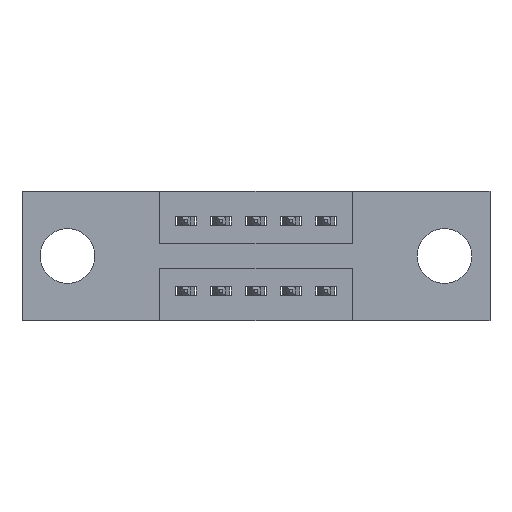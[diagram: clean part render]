
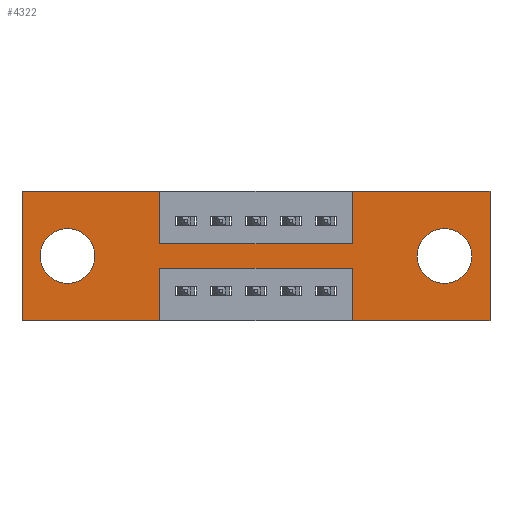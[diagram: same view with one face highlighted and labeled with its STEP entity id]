
A CAD part, front view. The second image highlights one B-rep face of the part: STEP entity #4322.
In plain terms, the highlighted planar face has unit normal (0, -1, 0).
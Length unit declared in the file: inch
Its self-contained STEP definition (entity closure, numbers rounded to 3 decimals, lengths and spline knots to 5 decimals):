
#21 = ORIENTED_EDGE ( 'NONE', *, *, #4895, .T. ) ;
#30 = CARTESIAN_POINT ( 'NONE',  ( 0.3925, 0., -0.22 ) ) ;
#129 = EDGE_CURVE ( 'NONE', #6393, #7987, #1377, .T. ) ;
#325 = CARTESIAN_POINT ( 'NONE',  ( 0.9425, 0., 0. ) ) ;
#330 = EDGE_LOOP ( 'NONE', ( #8569, #2305, #3220, #8067, #858, #7247, #7193, #8913, #1503, #1605, #1463, #5782 ) ) ;
#412 = CARTESIAN_POINT ( 'NONE',  ( 0., 0., 0. ) ) ;
#492 = CARTESIAN_POINT ( 'NONE',  ( 0.3925, 0., 0. ) ) ;
#537 = VERTEX_POINT ( 'NONE', #8299 ) ;
#549 = CARTESIAN_POINT ( 'NONE',  ( 1.205, 0., -0.185 ) ) ;
#681 = VECTOR ( 'NONE', #3747, 39.37008 ) ;
#836 = DIRECTION ( 'NONE',  ( 0., 0., 1. ) ) ;
#858 = ORIENTED_EDGE ( 'NONE', *, *, #2142, .F. ) ;
#921 = DIRECTION ( 'NONE',  ( 0., -1., 0. ) ) ;
#939 = LINE ( 'NONE', #3278, #3578 ) ;
#942 = VERTEX_POINT ( 'NONE', #8702 ) ;
#941 = CARTESIAN_POINT ( 'NONE',  ( 1.335, 0., 0. ) ) ;
#951 = VERTEX_POINT ( 'NONE', #3793 ) ;
#1284 = VERTEX_POINT ( 'NONE', #1442 ) ;
#1376 = DIRECTION ( 'NONE',  ( 0., 0., 1. ) ) ;
#1377 = CIRCLE ( 'NONE', #7139, 0.078 ) ;
#1381 = DIRECTION ( 'NONE',  ( 0., 1., 0. ) ) ;
#1442 = CARTESIAN_POINT ( 'NONE',  ( 0.3925, 0., -0.37 ) ) ;
#1462 = CARTESIAN_POINT ( 'NONE',  ( 0., 0., -0.37 ) ) ;
#1463 = ORIENTED_EDGE ( 'NONE', *, *, #4957, .F. ) ;
#1485 = CIRCLE ( 'NONE', #2098, 0.078 ) ;
#1503 = ORIENTED_EDGE ( 'NONE', *, *, #4004, .F. ) ;
#1540 = DIRECTION ( 'NONE',  ( -1., 0., 0. ) ) ;
#1567 = CARTESIAN_POINT ( 'NONE',  ( 0., 0., 0. ) ) ;
#1605 = ORIENTED_EDGE ( 'NONE', *, *, #7184, .F. ) ;
#1624 = VERTEX_POINT ( 'NONE', #7976 ) ;
#1632 = CARTESIAN_POINT ( 'NONE',  ( 0., 0., -0.37 ) ) ;
#1785 = DIRECTION ( 'NONE',  ( 0., 0., 1. ) ) ;
#1893 = VECTOR ( 'NONE', #1540, 39.37008 ) ;
#1915 = VECTOR ( 'NONE', #8106, 39.37008 ) ;
#1923 = LINE ( 'NONE', #492, #2034 ) ;
#2034 = VECTOR ( 'NONE', #3355, 39.37008 ) ;
#2061 = ORIENTED_EDGE ( 'NONE', *, *, #8958, .T. ) ;
#2098 = AXIS2_PLACEMENT_3D ( 'NONE', #549, #3452, #4260 ) ;
#2142 = EDGE_CURVE ( 'NONE', #6034, #8448, #7438, .T. ) ;
#2206 = LINE ( 'NONE', #5920, #1893 ) ;
#2228 = EDGE_CURVE ( 'NONE', #537, #8340, #939, .T. ) ;
#2305 = ORIENTED_EDGE ( 'NONE', *, *, #8248, .F. ) ;
#2360 = CIRCLE ( 'NONE', #3560, 0.078 ) ;
#2430 = LINE ( 'NONE', #7392, #681 ) ;
#2515 = VECTOR ( 'NONE', #7956, 39.37008 ) ;
#2756 = CARTESIAN_POINT ( 'NONE',  ( 0.13, 0., -0.263 ) ) ;
#2814 = VERTEX_POINT ( 'NONE', #1567 ) ;
#2815 = CARTESIAN_POINT ( 'NONE',  ( 0.13, 0., -0.185 ) ) ;
#2927 = CARTESIAN_POINT ( 'NONE',  ( 0., 0., 0. ) ) ;
#2930 = DIRECTION ( 'NONE',  ( -1., 0., 0. ) ) ;
#2950 = ORIENTED_EDGE ( 'NONE', *, *, #8917, .T. ) ;
#3128 = LINE ( 'NONE', #30, #8247 ) ;
#3137 = VECTOR ( 'NONE', #3843, 39.37008 ) ;
#3170 = CARTESIAN_POINT ( 'NONE',  ( 0.9425, 0., -0.37 ) ) ;
#3220 = ORIENTED_EDGE ( 'NONE', *, *, #8745, .F. ) ;
#3278 = CARTESIAN_POINT ( 'NONE',  ( 0.9425, 0., 0. ) ) ;
#3289 = EDGE_LOOP ( 'NONE', ( #21, #7867 ) ) ;
#3338 = FACE_BOUND ( 'NONE', #4185, .T. ) ;
#3355 = DIRECTION ( 'NONE',  ( 0., 0., -1. ) ) ;
#3452 = DIRECTION ( 'NONE',  ( 0., 1., 0. ) ) ;
#3480 = DIRECTION ( 'NONE',  ( 0., 1., 0. ) ) ;
#3560 = AXIS2_PLACEMENT_3D ( 'NONE', #2815, #5616, #4859 ) ;
#3578 = VECTOR ( 'NONE', #6212, 39.37008 ) ;
#3654 = CARTESIAN_POINT ( 'NONE',  ( 0.3925, 0., -0.15 ) ) ;
#3655 = LINE ( 'NONE', #1462, #1915 ) ;
#3747 = DIRECTION ( 'NONE',  ( 0., 0., -1. ) ) ;
#3749 = CARTESIAN_POINT ( 'NONE',  ( 1.205, 0., -0.263 ) ) ;
#3793 = CARTESIAN_POINT ( 'NONE',  ( 0.13, 0., -0.107 ) ) ;
#3843 = DIRECTION ( 'NONE',  ( 0., 0., -1. ) ) ;
#3879 = AXIS2_PLACEMENT_3D ( 'NONE', #1632, #921, #6011 ) ;
#4004 = EDGE_CURVE ( 'NONE', #7439, #4518, #1923, .T. ) ;
#4010 = VECTOR ( 'NONE', #6074, 39.37008 ) ;
#4168 = CARTESIAN_POINT ( 'NONE',  ( 1.205, 0., -0.107 ) ) ;
#4185 = EDGE_LOOP ( 'NONE', ( #2061, #2950 ) ) ;
#4260 = DIRECTION ( 'NONE',  ( 0., 0., -1. ) ) ;
#4322 = ADVANCED_FACE ( 'NONE', ( #6970, #3338, #7007 ), #8125, .T. ) ;
#4472 = EDGE_CURVE ( 'NONE', #4518, #537, #8663, .T. ) ;
#4518 = VERTEX_POINT ( 'NONE', #3654 ) ;
#4593 = EDGE_CURVE ( 'NONE', #942, #1284, #2430, .T. ) ;
#4692 = LINE ( 'NONE', #412, #4010 ) ;
#4778 = CIRCLE ( 'NONE', #5235, 0.078 ) ;
#4821 = DIRECTION ( 'NONE',  ( 1., 0., 0. ) ) ;
#4859 = DIRECTION ( 'NONE',  ( 0., 0., 1. ) ) ;
#4895 = EDGE_CURVE ( 'NONE', #7987, #6393, #1485, .T. ) ;
#4957 = EDGE_CURVE ( 'NONE', #1624, #2814, #7992, .T. ) ;
#5235 = AXIS2_PLACEMENT_3D ( 'NONE', #5519, #3480, #1376 ) ;
#5519 = CARTESIAN_POINT ( 'NONE',  ( 0.13, 0., -0.185 ) ) ;
#5532 = CARTESIAN_POINT ( 'NONE',  ( 0., 0., 0. ) ) ;
#5616 = DIRECTION ( 'NONE',  ( 0., 1., 0. ) ) ;
#5618 = VERTEX_POINT ( 'NONE', #9008 ) ;
#5782 = ORIENTED_EDGE ( 'NONE', *, *, #6403, .F. ) ;
#5920 = CARTESIAN_POINT ( 'NONE',  ( 0., 0., -0.37 ) ) ;
#6011 = DIRECTION ( 'NONE',  ( 0., 0., -1. ) ) ;
#6034 = VERTEX_POINT ( 'NONE', #6048 ) ;
#6048 = CARTESIAN_POINT ( 'NONE',  ( 1.335, 0., 0. ) ) ;
#6074 = DIRECTION ( 'NONE',  ( 1., 0., 0. ) ) ;
#6212 = DIRECTION ( 'NONE',  ( 0., 0., 1. ) ) ;
#6332 = CARTESIAN_POINT ( 'NONE',  ( 1.335, 0., -0.37 ) ) ;
#6360 = VERTEX_POINT ( 'NONE', #2756 ) ;
#6393 = VERTEX_POINT ( 'NONE', #3749 ) ;
#6403 = EDGE_CURVE ( 'NONE', #1284, #1624, #3655, .T. ) ;
#6587 = VECTOR ( 'NONE', #1785, 39.37008 ) ;
#6622 = VECTOR ( 'NONE', #4821, 39.37008 ) ;
#6732 = CARTESIAN_POINT ( 'NONE',  ( 0.9425, 0., -0.37 ) ) ;
#6970 = FACE_BOUND ( 'NONE', #3289, .T. ) ;
#7007 = FACE_OUTER_BOUND ( 'NONE', #330, .T. ) ;
#7139 = AXIS2_PLACEMENT_3D ( 'NONE', #8025, #1381, #7974 ) ;
#7184 = EDGE_CURVE ( 'NONE', #2814, #7439, #8417, .T. ) ;
#7193 = ORIENTED_EDGE ( 'NONE', *, *, #2228, .F. ) ;
#7247 = ORIENTED_EDGE ( 'NONE', *, *, #8352, .F. ) ;
#7392 = CARTESIAN_POINT ( 'NONE',  ( 0.3925, 0., -0.37 ) ) ;
#7439 = VERTEX_POINT ( 'NONE', #8883 ) ;
#7438 = LINE ( 'NONE', #941, #3137 ) ;
#7729 = VERTEX_POINT ( 'NONE', #6732 ) ;
#7766 = CARTESIAN_POINT ( 'NONE',  ( 0.3925, 0., -0.15 ) ) ;
#7867 = ORIENTED_EDGE ( 'NONE', *, *, #129, .T. ) ;
#7956 = DIRECTION ( 'NONE',  ( 1., 0., 0. ) ) ;
#7974 = DIRECTION ( 'NONE',  ( 0., 0., -1. ) ) ;
#7976 = CARTESIAN_POINT ( 'NONE',  ( 0., 0., -0.37 ) ) ;
#7987 = VERTEX_POINT ( 'NONE', #4168 ) ;
#7992 = LINE ( 'NONE', #2927, #7995 ) ;
#7995 = VECTOR ( 'NONE', #836, 39.37008 ) ;
#8025 = CARTESIAN_POINT ( 'NONE',  ( 1.205, 0., -0.185 ) ) ;
#8067 = ORIENTED_EDGE ( 'NONE', *, *, #8564, .F. ) ;
#8106 = DIRECTION ( 'NONE',  ( -1., 0., 0. ) ) ;
#8125 = PLANE ( 'NONE',  #3879 ) ;
#8247 = VECTOR ( 'NONE', #2930, 39.37008 ) ;
#8248 = EDGE_CURVE ( 'NONE', #5618, #942, #3128, .T. ) ;
#8299 = CARTESIAN_POINT ( 'NONE',  ( 0.9425, 0., -0.15 ) ) ;
#8340 = VERTEX_POINT ( 'NONE', #325 ) ;
#8352 = EDGE_CURVE ( 'NONE', #8340, #6034, #4692, .T. ) ;
#8417 = LINE ( 'NONE', #5532, #6622 ) ;
#8448 = VERTEX_POINT ( 'NONE', #6332 ) ;
#8564 = EDGE_CURVE ( 'NONE', #8448, #7729, #2206, .T. ) ;
#8569 = ORIENTED_EDGE ( 'NONE', *, *, #4593, .F. ) ;
#8663 = LINE ( 'NONE', #7766, #2515 ) ;
#8702 = CARTESIAN_POINT ( 'NONE',  ( 0.3925, 0., -0.22 ) ) ;
#8745 = EDGE_CURVE ( 'NONE', #7729, #5618, #8885, .T. ) ;
#8883 = CARTESIAN_POINT ( 'NONE',  ( 0.3925, 0., 0. ) ) ;
#8885 = LINE ( 'NONE', #3170, #6587 ) ;
#8913 = ORIENTED_EDGE ( 'NONE', *, *, #4472, .F. ) ;
#8917 = EDGE_CURVE ( 'NONE', #6360, #951, #4778, .T. ) ;
#8958 = EDGE_CURVE ( 'NONE', #951, #6360, #2360, .T. ) ;
#9008 = CARTESIAN_POINT ( 'NONE',  ( 0.9425, 0., -0.22 ) ) ;
